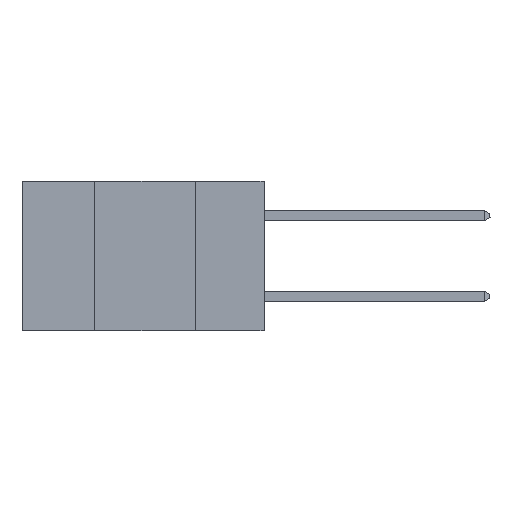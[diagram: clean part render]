
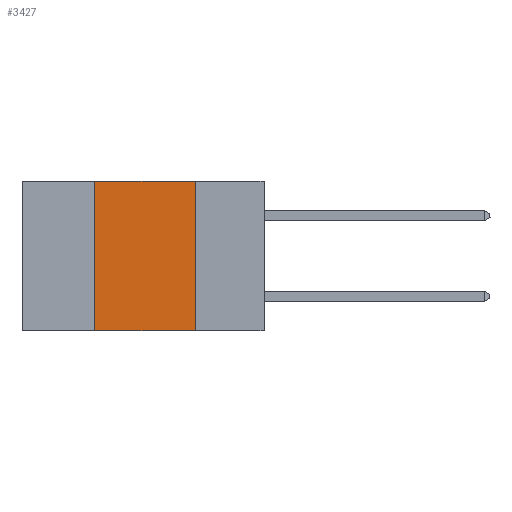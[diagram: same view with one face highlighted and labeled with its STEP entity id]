
A CAD part, left-side view. The second image highlights one B-rep face of the part: STEP entity #3427.
In plain terms, the highlighted planar face has unit normal (-1, 0, 0).
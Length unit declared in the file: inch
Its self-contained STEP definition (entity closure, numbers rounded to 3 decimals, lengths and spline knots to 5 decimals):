
#1030 = CARTESIAN_POINT ( 'NONE',  ( 0., 0.6, 0. ) ) ;
#1423 = DIRECTION ( 'NONE',  ( 0., 0., -1. ) ) ;
#1742 = LINE ( 'NONE', #1030, #6786 ) ;
#2678 = LINE ( 'NONE', #18938, #3443 ) ;
#2688 = EDGE_CURVE ( 'NONE', #8403, #5996, #27080, .T. ) ;
#3427 = ADVANCED_FACE ( 'NONE', ( #21936 ), #11131, .F. ) ;
#3443 = VECTOR ( 'NONE', #31260, 39.37008 ) ;
#5996 = VERTEX_POINT ( 'NONE', #17731 ) ;
#6786 = VECTOR ( 'NONE', #10519, 39.37008 ) ;
#7064 = ORIENTED_EDGE ( 'NONE', *, *, #18859, .T. ) ;
#8403 = VERTEX_POINT ( 'NONE', #31181 ) ;
#10338 = CARTESIAN_POINT ( 'NONE',  ( 0., 0.6, -0.37 ) ) ;
#10519 = DIRECTION ( 'NONE',  ( 0., -1., 0. ) ) ;
#10982 = VERTEX_POINT ( 'NONE', #29024 ) ;
#11131 = PLANE ( 'NONE',  #12856 ) ;
#12281 = DIRECTION ( 'NONE',  ( 0., 0., -1. ) ) ;
#12696 = DIRECTION ( 'NONE',  ( 0., -1., 0. ) ) ;
#12856 = AXIS2_PLACEMENT_3D ( 'NONE', #31009, #16084, #1423 ) ;
#14269 = VERTEX_POINT ( 'NONE', #17902 ) ;
#14478 = ORIENTED_EDGE ( 'NONE', *, *, #20271, .F. ) ;
#16084 = DIRECTION ( 'NONE',  ( 1., 0., 0. ) ) ;
#17731 = CARTESIAN_POINT ( 'NONE',  ( 0., 0.17, -0.37 ) ) ;
#17902 = CARTESIAN_POINT ( 'NONE',  ( 0., 0.42, -0.37 ) ) ;
#18859 = EDGE_CURVE ( 'NONE', #14269, #5996, #31493, .T. ) ;
#18938 = CARTESIAN_POINT ( 'NONE',  ( 0., 0.42, 0. ) ) ;
#19305 = CARTESIAN_POINT ( 'NONE',  ( 0., 0.17, 0. ) ) ;
#20032 = VECTOR ( 'NONE', #12281, 39.37008 ) ;
#20271 = EDGE_CURVE ( 'NONE', #14269, #10982, #2678, .T. ) ;
#21102 = EDGE_LOOP ( 'NONE', ( #23588, #26193, #14478, #7064 ) ) ;
#21936 = FACE_OUTER_BOUND ( 'NONE', #21102, .T. ) ;
#23313 = VECTOR ( 'NONE', #12696, 39.37008 ) ;
#23483 = EDGE_CURVE ( 'NONE', #10982, #8403, #1742, .T. ) ;
#23588 = ORIENTED_EDGE ( 'NONE', *, *, #2688, .F. ) ;
#26193 = ORIENTED_EDGE ( 'NONE', *, *, #23483, .F. ) ;
#27080 = LINE ( 'NONE', #19305, #20032 ) ;
#29024 = CARTESIAN_POINT ( 'NONE',  ( 0., 0.42, 0. ) ) ;
#31009 = CARTESIAN_POINT ( 'NONE',  ( 0., 0.6, 0. ) ) ;
#31181 = CARTESIAN_POINT ( 'NONE',  ( 0., 0.17, 0. ) ) ;
#31260 = DIRECTION ( 'NONE',  ( 0., 0., 1. ) ) ;
#31493 = LINE ( 'NONE', #10338, #23313 ) ;
